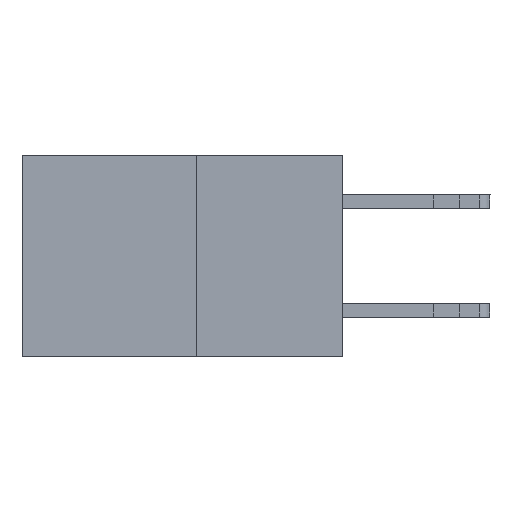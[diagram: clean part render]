
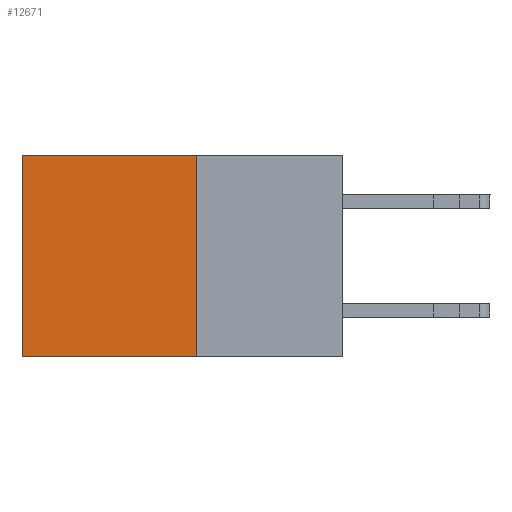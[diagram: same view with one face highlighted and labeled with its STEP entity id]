
A CAD part, left-side view. The second image highlights one B-rep face of the part: STEP entity #12671.
In plain terms, the highlighted planar face has unit normal (-1, 0, 0).
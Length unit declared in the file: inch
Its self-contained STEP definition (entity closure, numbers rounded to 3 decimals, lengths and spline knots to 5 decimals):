
#1031 = CARTESIAN_POINT ( 'NONE',  ( 0.277, 0.27, -0.37 ) ) ;
#1142 = VERTEX_POINT ( 'NONE', #17349 ) ;
#1314 = VERTEX_POINT ( 'NONE', #21895 ) ;
#2986 = ORIENTED_EDGE ( 'NONE', *, *, #21434, .F. ) ;
#3679 = VECTOR ( 'NONE', #17024, 39.37008 ) ;
#4575 = DIRECTION ( 'NONE',  ( 0., 1., 0. ) ) ;
#4604 = EDGE_CURVE ( 'NONE', #1314, #1142, #21080, .T. ) ;
#6764 = ORIENTED_EDGE ( 'NONE', *, *, #4604, .T. ) ;
#7783 = VECTOR ( 'NONE', #21977, 39.37008 ) ;
#8058 = VERTEX_POINT ( 'NONE', #13545 ) ;
#8259 = FACE_OUTER_BOUND ( 'NONE', #14763, .T. ) ;
#9906 = ORIENTED_EDGE ( 'NONE', *, *, #13584, .F. ) ;
#9983 = CARTESIAN_POINT ( 'NONE',  ( 0.277, 0.27, 0. ) ) ;
#11867 = VECTOR ( 'NONE', #4575, 39.37008 ) ;
#12671 = ADVANCED_FACE ( 'NONE', ( #8259 ), #16729, .F. ) ;
#13227 = EDGE_CURVE ( 'NONE', #22815, #1314, #20057, .T. ) ;
#13545 = CARTESIAN_POINT ( 'NONE',  ( 0.277, 0.27, -0.37 ) ) ;
#13584 = EDGE_CURVE ( 'NONE', #8058, #1142, #16784, .T. ) ;
#14763 = EDGE_LOOP ( 'NONE', ( #6764, #9906, #2986, #16694 ) ) ;
#15646 = AXIS2_PLACEMENT_3D ( 'NONE', #1031, #18681, #18570 ) ;
#16441 = CARTESIAN_POINT ( 'NONE',  ( 0.277, 0.27, -0.37 ) ) ;
#16694 = ORIENTED_EDGE ( 'NONE', *, *, #13227, .T. ) ;
#16729 = PLANE ( 'NONE',  #15646 ) ;
#16784 = LINE ( 'NONE', #18406, #11867 ) ;
#17024 = DIRECTION ( 'NONE',  ( 0., 1., 0. ) ) ;
#17119 = CARTESIAN_POINT ( 'NONE',  ( 0.277, 0.27, 0. ) ) ;
#17349 = CARTESIAN_POINT ( 'NONE',  ( 0.277, 0.59, -0.37 ) ) ;
#17383 = DIRECTION ( 'NONE',  ( 0., 0., -1. ) ) ;
#18169 = LINE ( 'NONE', #16441, #7783 ) ;
#18406 = CARTESIAN_POINT ( 'NONE',  ( 0.277, 0.27, -0.37 ) ) ;
#18570 = DIRECTION ( 'NONE',  ( 0., 0., -1. ) ) ;
#18681 = DIRECTION ( 'NONE',  ( 1., 0., 0. ) ) ;
#19572 = CARTESIAN_POINT ( 'NONE',  ( 0.277, 0.59, -0.37 ) ) ;
#20057 = LINE ( 'NONE', #9983, #3679 ) ;
#21080 = LINE ( 'NONE', #19572, #22210 ) ;
#21434 = EDGE_CURVE ( 'NONE', #22815, #8058, #18169, .T. ) ;
#21895 = CARTESIAN_POINT ( 'NONE',  ( 0.277, 0.59, 0. ) ) ;
#21977 = DIRECTION ( 'NONE',  ( 0., 0., -1. ) ) ;
#22210 = VECTOR ( 'NONE', #17383, 39.37008 ) ;
#22815 = VERTEX_POINT ( 'NONE', #17119 ) ;
